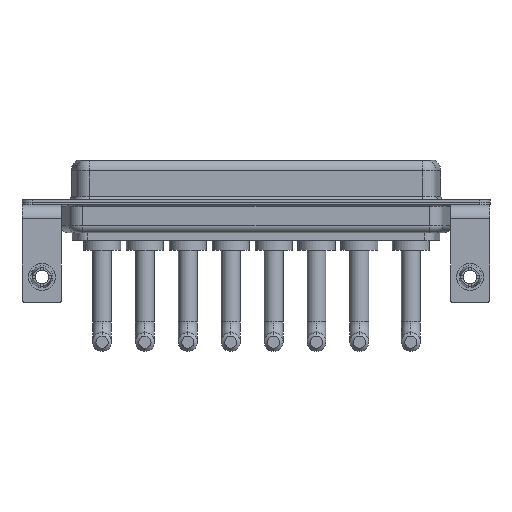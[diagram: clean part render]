
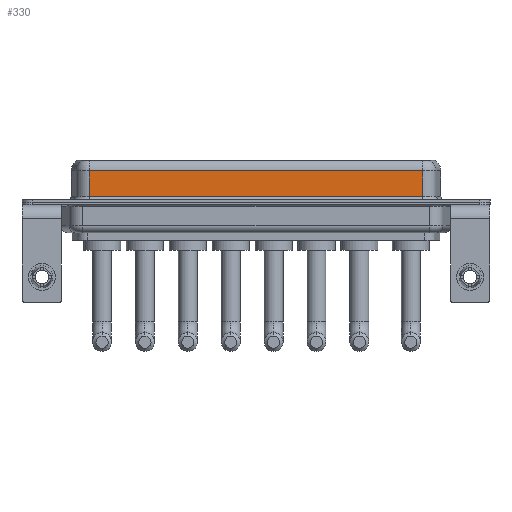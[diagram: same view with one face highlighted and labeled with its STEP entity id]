
A CAD part, front view. The second image highlights one B-rep face of the part: STEP entity #330.
In plain terms, the highlighted planar face has unit normal (0, -1, 0).
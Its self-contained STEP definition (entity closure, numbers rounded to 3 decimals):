
#330 = ADVANCED_FACE ( 'NONE', ( #13134 ), #1315, .F. ) ;
#590 = VECTOR ( 'NONE', #6312, 1000. ) ;
#790 = CARTESIAN_POINT ( 'NONE',  ( 56.462, -3.95, 0.9 ) ) ;
#1315 = PLANE ( 'NONE',  #14231 ) ;
#1790 = CARTESIAN_POINT ( 'NONE',  ( 56.462, -3.95, 0.9 ) ) ;
#2253 = DIRECTION ( 'NONE',  ( 0., 0., -1. ) ) ;
#2360 = VERTEX_POINT ( 'NONE', #11122 ) ;
#2397 = DIRECTION ( 'NONE',  ( 0., 0., -1. ) ) ;
#2519 = EDGE_LOOP ( 'NONE', ( #11902, #6026, #12602, #11987 ) ) ;
#2746 = EDGE_CURVE ( 'NONE', #2360, #10263, #3497, .T. ) ;
#3497 = LINE ( 'NONE', #9668, #8762 ) ;
#3690 = DIRECTION ( 'NONE',  ( 0., 0., 1. ) ) ;
#4250 = LINE ( 'NONE', #1790, #590 ) ;
#6026 = ORIENTED_EDGE ( 'NONE', *, *, #11668, .T. ) ;
#6312 = DIRECTION ( 'NONE',  ( 1., 0., 0. ) ) ;
#7959 = VECTOR ( 'NONE', #2253, 1000. ) ;
#8581 = CARTESIAN_POINT ( 'NONE',  ( 56.462, -3.95, 4.65 ) ) ;
#8762 = VECTOR ( 'NONE', #2397, 1000. ) ;
#9668 = CARTESIAN_POINT ( 'NONE',  ( 7.038, -3.95, 6.4 ) ) ;
#10025 = VERTEX_POINT ( 'NONE', #10398 ) ;
#10263 = VERTEX_POINT ( 'NONE', #12797 ) ;
#10398 = CARTESIAN_POINT ( 'NONE',  ( 56.462, -3.95, 4.65 ) ) ;
#11042 = LINE ( 'NONE', #8581, #12495 ) ;
#11122 = CARTESIAN_POINT ( 'NONE',  ( 7.038, -3.95, 4.65 ) ) ;
#11385 = EDGE_CURVE ( 'NONE', #10263, #13258, #4250, .T. ) ;
#11668 = EDGE_CURVE ( 'NONE', #10025, #2360, #11042, .T. ) ;
#11902 = ORIENTED_EDGE ( 'NONE', *, *, #13017, .F. ) ;
#11987 = ORIENTED_EDGE ( 'NONE', *, *, #11385, .T. ) ;
#11991 = CARTESIAN_POINT ( 'NONE',  ( 56.462, -3.95, 6.4 ) ) ;
#12255 = CARTESIAN_POINT ( 'NONE',  ( 56.462, -3.95, 6.4 ) ) ;
#12495 = VECTOR ( 'NONE', #13125, 1000. ) ;
#12602 = ORIENTED_EDGE ( 'NONE', *, *, #2746, .T. ) ;
#12797 = CARTESIAN_POINT ( 'NONE',  ( 7.038, -3.95, 0.9 ) ) ;
#13017 = EDGE_CURVE ( 'NONE', #10025, #13258, #13118, .T. ) ;
#13118 = LINE ( 'NONE', #11991, #7959 ) ;
#13125 = DIRECTION ( 'NONE',  ( -1., 0., 0. ) ) ;
#13134 = FACE_OUTER_BOUND ( 'NONE', #2519, .T. ) ;
#13258 = VERTEX_POINT ( 'NONE', #790 ) ;
#14231 = AXIS2_PLACEMENT_3D ( 'NONE', #12255, #15678, #3690 ) ;
#15678 = DIRECTION ( 'NONE',  ( 0., 1., 0. ) ) ;
